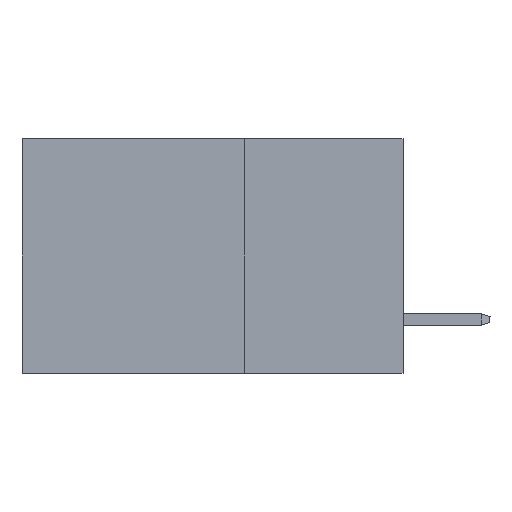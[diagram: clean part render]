
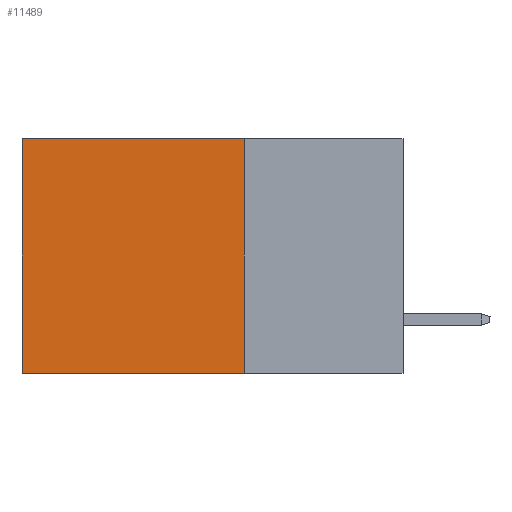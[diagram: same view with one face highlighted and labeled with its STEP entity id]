
A CAD part, left-side view. The second image highlights one B-rep face of the part: STEP entity #11489.
In plain terms, the highlighted planar face has unit normal (-1, 0, 0).
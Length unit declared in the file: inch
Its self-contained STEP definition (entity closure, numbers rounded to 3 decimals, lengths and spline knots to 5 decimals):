
#267 = VERTEX_POINT ( 'NONE', #14128 ) ;
#2033 = DIRECTION ( 'NONE',  ( 0., 0., -1. ) ) ;
#3095 = CARTESIAN_POINT ( 'NONE',  ( 0.2875, 0.25, 0. ) ) ;
#3901 = ORIENTED_EDGE ( 'NONE', *, *, #40614, .T. ) ;
#4778 = ORIENTED_EDGE ( 'NONE', *, *, #32866, .T. ) ;
#6106 = LINE ( 'NONE', #35025, #47834 ) ;
#9458 = PLANE ( 'NONE',  #10263 ) ;
#10263 = AXIS2_PLACEMENT_3D ( 'NONE', #42800, #16147, #12441 ) ;
#10859 = VERTEX_POINT ( 'NONE', #26298 ) ;
#11489 = ADVANCED_FACE ( 'NONE', ( #27875 ), #9458, .F. ) ;
#12441 = DIRECTION ( 'NONE',  ( 0., 0., -1. ) ) ;
#12620 = EDGE_CURVE ( 'NONE', #267, #19420, #39222, .T. ) ;
#14128 = CARTESIAN_POINT ( 'NONE',  ( 0.2875, 0.25, 0. ) ) ;
#15675 = CARTESIAN_POINT ( 'NONE',  ( 0.2875, 0.25, -0.37 ) ) ;
#16147 = DIRECTION ( 'NONE',  ( 1., 0., 0. ) ) ;
#17708 = DIRECTION ( 'NONE',  ( 0., 0., -1. ) ) ;
#19420 = VERTEX_POINT ( 'NONE', #15675 ) ;
#21095 = DIRECTION ( 'NONE',  ( 0., 1., 0. ) ) ;
#21829 = CARTESIAN_POINT ( 'NONE',  ( 0.2875, 0.6, 0. ) ) ;
#21935 = VECTOR ( 'NONE', #21940, 39.37008 ) ;
#21940 = DIRECTION ( 'NONE',  ( 0., 1., 0. ) ) ;
#23595 = CARTESIAN_POINT ( 'NONE',  ( 0.2875, 0.25, 0. ) ) ;
#25267 = CARTESIAN_POINT ( 'NONE',  ( 0.2875, 0.6, 0. ) ) ;
#25749 = EDGE_LOOP ( 'NONE', ( #3901, #46909, #35239, #4778 ) ) ;
#26298 = CARTESIAN_POINT ( 'NONE',  ( 0.2875, 0.6, -0.37 ) ) ;
#27875 = FACE_OUTER_BOUND ( 'NONE', #25749, .T. ) ;
#29036 = VERTEX_POINT ( 'NONE', #21829 ) ;
#29999 = LINE ( 'NONE', #3095, #21935 ) ;
#30919 = VECTOR ( 'NONE', #17708, 39.37008 ) ;
#32866 = EDGE_CURVE ( 'NONE', #267, #29036, #29999, .T. ) ;
#34151 = EDGE_CURVE ( 'NONE', #19420, #10859, #6106, .T. ) ;
#35025 = CARTESIAN_POINT ( 'NONE',  ( 0.2875, 0.25, -0.37 ) ) ;
#35239 = ORIENTED_EDGE ( 'NONE', *, *, #12620, .F. ) ;
#36265 = LINE ( 'NONE', #25267, #30919 ) ;
#39222 = LINE ( 'NONE', #23595, #46369 ) ;
#40614 = EDGE_CURVE ( 'NONE', #29036, #10859, #36265, .T. ) ;
#42800 = CARTESIAN_POINT ( 'NONE',  ( 0.2875, 0.25, 0. ) ) ;
#46369 = VECTOR ( 'NONE', #2033, 39.37008 ) ;
#46909 = ORIENTED_EDGE ( 'NONE', *, *, #34151, .F. ) ;
#47834 = VECTOR ( 'NONE', #21095, 39.37008 ) ;
